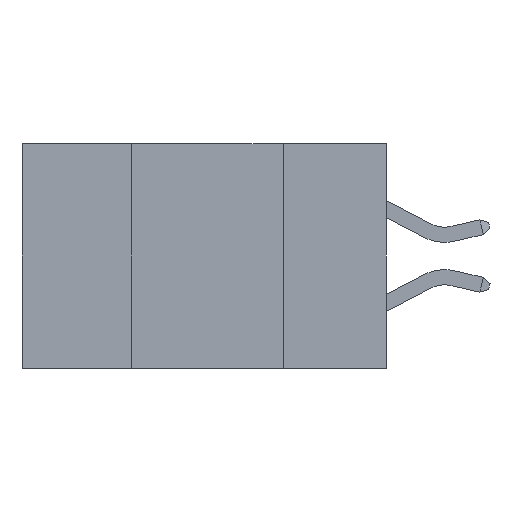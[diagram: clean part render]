
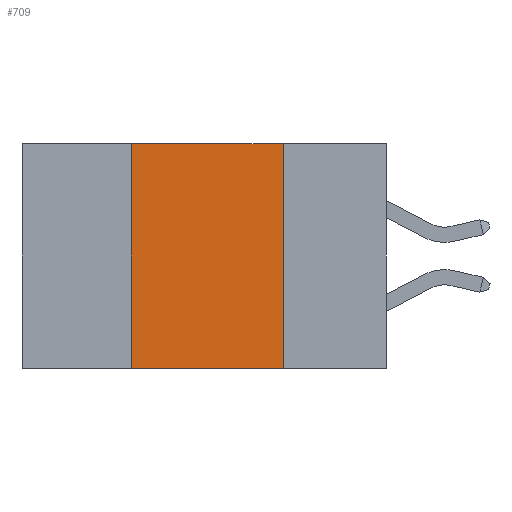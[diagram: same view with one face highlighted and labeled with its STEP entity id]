
A CAD part, left-side view. The second image highlights one B-rep face of the part: STEP entity #709.
In plain terms, the highlighted planar face has unit normal (-1, 0, 0).
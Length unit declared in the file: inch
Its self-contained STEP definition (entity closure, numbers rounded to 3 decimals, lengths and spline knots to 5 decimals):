
#3 = ORIENTED_EDGE ( 'NONE', *, *, #8975, .T. ) ;
#328 = DIRECTION ( 'NONE',  ( 0., -1., 0. ) ) ;
#422 = CARTESIAN_POINT ( 'NONE',  ( 0., 0.42, 0. ) ) ;
#709 = ADVANCED_FACE ( 'NONE', ( #3727 ), #6692, .F. ) ;
#930 = CARTESIAN_POINT ( 'NONE',  ( 0., 0.17, -0.37 ) ) ;
#1299 = ORIENTED_EDGE ( 'NONE', *, *, #4275, .F. ) ;
#1937 = EDGE_CURVE ( 'NONE', #7662, #8169, #5529, .T. ) ;
#1955 = DIRECTION ( 'NONE',  ( 0., -1., 0. ) ) ;
#2030 = ORIENTED_EDGE ( 'NONE', *, *, #1937, .F. ) ;
#2526 = AXIS2_PLACEMENT_3D ( 'NONE', #7751, #3066, #7591 ) ;
#2553 = VECTOR ( 'NONE', #8171, 39.37008 ) ;
#2969 = LINE ( 'NONE', #5959, #4535 ) ;
#3066 = DIRECTION ( 'NONE',  ( 1., 0., 0. ) ) ;
#3404 = LINE ( 'NONE', #8082, #2553 ) ;
#3727 = FACE_OUTER_BOUND ( 'NONE', #8777, .T. ) ;
#4275 = EDGE_CURVE ( 'NONE', #7461, #7662, #3404, .T. ) ;
#4535 = VECTOR ( 'NONE', #6787, 39.37008 ) ;
#4813 = VECTOR ( 'NONE', #328, 39.37008 ) ;
#5436 = VERTEX_POINT ( 'NONE', #930 ) ;
#5529 = LINE ( 'NONE', #7611, #4813 ) ;
#5748 = VECTOR ( 'NONE', #1955, 39.37008 ) ;
#5959 = CARTESIAN_POINT ( 'NONE',  ( 0., 0.17, -0.37 ) ) ;
#6233 = CARTESIAN_POINT ( 'NONE',  ( 0., 0.17, 0. ) ) ;
#6526 = CARTESIAN_POINT ( 'NONE',  ( 0., 0.6, -0.37 ) ) ;
#6692 = PLANE ( 'NONE',  #2526 ) ;
#6787 = DIRECTION ( 'NONE',  ( 0., 0., -1. ) ) ;
#7461 = VERTEX_POINT ( 'NONE', #8040 ) ;
#7591 = DIRECTION ( 'NONE',  ( 0., 0., -1. ) ) ;
#7611 = CARTESIAN_POINT ( 'NONE',  ( 0., 0.6, 0. ) ) ;
#7620 = ORIENTED_EDGE ( 'NONE', *, *, #9195, .F. ) ;
#7662 = VERTEX_POINT ( 'NONE', #422 ) ;
#7751 = CARTESIAN_POINT ( 'NONE',  ( 0., 0.6, 0. ) ) ;
#8040 = CARTESIAN_POINT ( 'NONE',  ( 0., 0.42, -0.37 ) ) ;
#8082 = CARTESIAN_POINT ( 'NONE',  ( 0., 0.42, -0.37 ) ) ;
#8169 = VERTEX_POINT ( 'NONE', #6233 ) ;
#8171 = DIRECTION ( 'NONE',  ( 0., 0., 1. ) ) ;
#8777 = EDGE_LOOP ( 'NONE', ( #7620, #2030, #1299, #3 ) ) ;
#8975 = EDGE_CURVE ( 'NONE', #7461, #5436, #11361, .T. ) ;
#9195 = EDGE_CURVE ( 'NONE', #8169, #5436, #2969, .T. ) ;
#11361 = LINE ( 'NONE', #6526, #5748 ) ;
